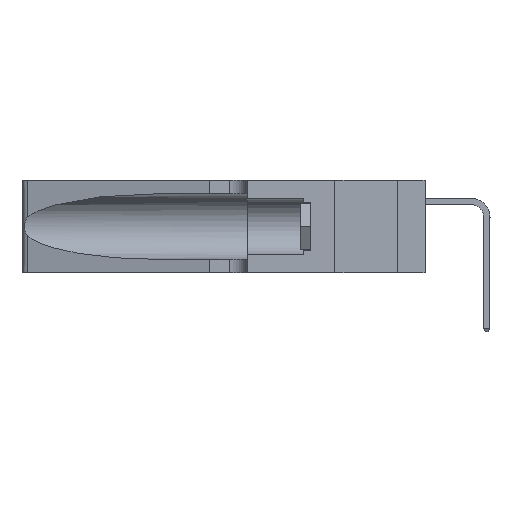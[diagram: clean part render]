
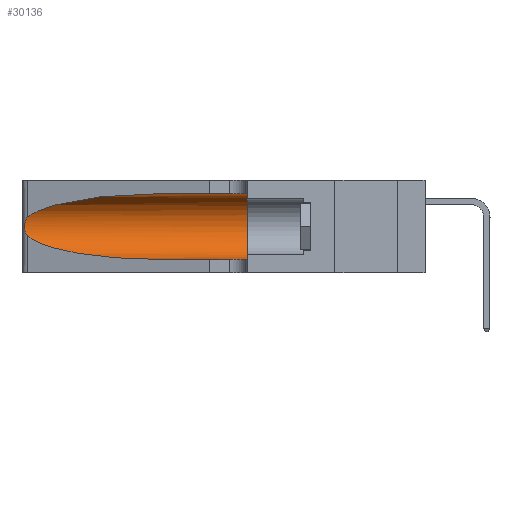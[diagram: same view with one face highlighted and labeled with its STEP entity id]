
A CAD part, left-side view. The second image highlights one B-rep face of the part: STEP entity #30136.
In plain terms, the highlighted cylindrical face has radius 3.308 mm (diameter 6.617 mm), a partial arc.
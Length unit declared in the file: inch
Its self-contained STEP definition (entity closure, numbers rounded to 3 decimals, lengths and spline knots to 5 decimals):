
#444 = CARTESIAN_POINT ( 'NONE',  ( 0.25555, 1.22994, 0.2215 ) ) ;
#615 = CARTESIAN_POINT ( 'NONE',  ( 0.25487, 1.22718, 0.14631 ) ) ;
#868 = VERTEX_POINT ( 'NONE', #48752 ) ;
#929 = DIRECTION ( 'NONE',  ( 0., -1., 0. ) ) ;
#1333 = FACE_OUTER_BOUND ( 'NONE', #9820, .T. ) ;
#1765 = CARTESIAN_POINT ( 'NONE',  ( 0.1305, 0.72297, 0.31525 ) ) ;
#2274 = CARTESIAN_POINT ( 'NONE',  ( 0.1305, 1.61858, 0.31525 ) ) ;
#4525 = CARTESIAN_POINT ( 'NONE',  ( 0.25487, 1.22718, 0.22369 ) ) ;
#4927 = DIRECTION ( 'NONE',  ( 0., -1., 0. ) ) ;
#5170 = ORIENTED_EDGE ( 'NONE', *, *, #38630, .F. ) ;
#5724 = CARTESIAN_POINT ( 'NONE',  ( 0.1305, 0.72297, 0.05475 ) ) ;
#6654 =( BOUNDED_CURVE ( )  B_SPLINE_CURVE ( 3, ( #50206, #21875, #30033, #5724 ),
 .UNSPECIFIED., .F., .F. ) 
 B_SPLINE_CURVE_WITH_KNOTS ( ( 4, 4 ),
 ( 3.44316, 4.71239 ),
 .UNSPECIFIED. ) 
 CURVE ( )  GEOMETRIC_REPRESENTATION_ITEM ( )  RATIONAL_B_SPLINE_CURVE ( ( 1., 0.87, 0.87, 1. ) ) 
 REPRESENTATION_ITEM ( '' )  );
#8615 = CARTESIAN_POINT ( 'NONE',  ( 0.25854, 1.2359, 0.20912 ) ) ;
#9820 = EDGE_LOOP ( 'NONE', ( #46603, #17279, #41911, #24127, #30519, #5170 ) ) ;
#12690 = CARTESIAN_POINT ( 'NONE',  ( 0.26075, 1.23896, 0.19203 ) ) ;
#12732 = CARTESIAN_POINT ( 'NONE',  ( 0.25487, 1.22718, 0.22369 ) ) ;
#14310 = CARTESIAN_POINT ( 'NONE',  ( 0.1305, 0.35, 0.185 ) ) ;
#14736 = CARTESIAN_POINT ( 'NONE',  ( 0.25487, 1.22718, 0.22369 ) ) ;
#16659 = CARTESIAN_POINT ( 'NONE',  ( 0.1305, 0.72297, 0.31525 ) ) ;
#16790 = CARTESIAN_POINT ( 'NONE',  ( 0.26017, 1.23833, 0.17102 ) ) ;
#17021 = VERTEX_POINT ( 'NONE', #27791 ) ;
#17165 = EDGE_CURVE ( 'NONE', #49533, #18717, #21082, .T. ) ;
#17279 = ORIENTED_EDGE ( 'NONE', *, *, #17165, .T. ) ;
#18390 = DIRECTION ( 'NONE',  ( 0., 0., 1. ) ) ;
#18717 = VERTEX_POINT ( 'NONE', #49147 ) ;
#18880 = EDGE_CURVE ( 'NONE', #18717, #28543, #6654, .T. ) ;
#20857 = CARTESIAN_POINT ( 'NONE',  ( 0.25789, 1.23486, 0.15765 ) ) ;
#21082 = B_SPLINE_CURVE_WITH_KNOTS ( 'NONE', 3,
 ( #4525, #444, #28835, #32958, #8615, #36999, #12690, #41062, #16790, #45137, #20857, #49196, #24958, #615 ),
 .UNSPECIFIED., .F., .F.,
 ( 4, 2, 2, 2, 2, 2, 4 ),
 ( 0., 0.00027, 0.00053, 0.00107, 0.0016, 0.00187, 0.00214 ),
 .UNSPECIFIED. ) ;
#21369 = DIRECTION ( 'NONE',  ( 0., 0., -1. ) ) ;
#21875 = CARTESIAN_POINT ( 'NONE',  ( 0.2373, 1.15595, 0.08982 ) ) ;
#24127 = ORIENTED_EDGE ( 'NONE', *, *, #34479, .T. ) ;
#24958 = CARTESIAN_POINT ( 'NONE',  ( 0.25555, 1.22993, 0.14849 ) ) ;
#25184 = CARTESIAN_POINT ( 'NONE',  ( 0.1305, 1.61858, 0.05475 ) ) ;
#27354 = CARTESIAN_POINT ( 'NONE',  ( 0.1305, 0.72297, 0.05475 ) ) ;
#27708 = EDGE_CURVE ( 'NONE', #868, #17021, #36431, .T. ) ;
#27791 = CARTESIAN_POINT ( 'NONE',  ( 0.1305, 0.35, 0.05475 ) ) ;
#28543 = VERTEX_POINT ( 'NONE', #27354 ) ;
#28835 = CARTESIAN_POINT ( 'NONE',  ( 0.25639, 1.23184, 0.21858 ) ) ;
#30033 = CARTESIAN_POINT ( 'NONE',  ( 0.18966, 0.96281, 0.05475 ) ) ;
#30136 = ADVANCED_FACE ( 'NONE', ( #1333 ), #32465, .F. ) ;
#30519 = ORIENTED_EDGE ( 'NONE', *, *, #27708, .F. ) ;
#32465 = CYLINDRICAL_SURFACE ( 'NONE', #32975, 0.13025 ) ;
#32958 = CARTESIAN_POINT ( 'NONE',  ( 0.25787, 1.23484, 0.2124 ) ) ;
#32975 = AXIS2_PLACEMENT_3D ( 'NONE', #45629, #929, #21369 ) ;
#34479 = EDGE_CURVE ( 'NONE', #28543, #17021, #41619, .T. ) ;
#34764 = DIRECTION ( 'NONE',  ( 0., -1., 0. ) ) ;
#36431 = CIRCLE ( 'NONE', #37283, 0.13025 ) ;
#36999 = CARTESIAN_POINT ( 'NONE',  ( 0.26018, 1.23835, 0.19895 ) ) ;
#37035 = CARTESIAN_POINT ( 'NONE',  ( 0.2373, 1.15595, 0.28018 ) ) ;
#37283 = AXIS2_PLACEMENT_3D ( 'NONE', #14310, #42680, #18390 ) ;
#38630 = EDGE_CURVE ( 'NONE', #47607, #868, #45646, .T. ) ;
#39789 =( BOUNDED_CURVE ( )  B_SPLINE_CURVE ( 3, ( #16659, #49061, #37035, #12732 ),
 .UNSPECIFIED., .F., .T. ) 
 B_SPLINE_CURVE_WITH_KNOTS ( ( 4, 4 ),
 ( 1.5708, 2.84003 ),
 .UNSPECIFIED. ) 
 CURVE ( )  GEOMETRIC_REPRESENTATION_ITEM ( )  RATIONAL_B_SPLINE_CURVE ( ( 1., 0.87, 0.87, 1. ) ) 
 REPRESENTATION_ITEM ( '' )  );
#41062 = CARTESIAN_POINT ( 'NONE',  ( 0.26075, 1.23896, 0.178 ) ) ;
#41619 = LINE ( 'NONE', #25184, #42911 ) ;
#41911 = ORIENTED_EDGE ( 'NONE', *, *, #18880, .T. ) ;
#42680 = DIRECTION ( 'NONE',  ( 0., 1., 0. ) ) ;
#42911 = VECTOR ( 'NONE', #4927, 39.37008 ) ;
#44386 = VECTOR ( 'NONE', #34764, 39.37008 ) ;
#45137 = CARTESIAN_POINT ( 'NONE',  ( 0.25856, 1.23593, 0.16098 ) ) ;
#45629 = CARTESIAN_POINT ( 'NONE',  ( 0.1305, 1.61858, 0.185 ) ) ;
#45646 = LINE ( 'NONE', #2274, #44386 ) ;
#46603 = ORIENTED_EDGE ( 'NONE', *, *, #46632, .T. ) ;
#46632 = EDGE_CURVE ( 'NONE', #47607, #49533, #39789, .T. ) ;
#47607 = VERTEX_POINT ( 'NONE', #1765 ) ;
#48752 = CARTESIAN_POINT ( 'NONE',  ( 0.1305, 0.35, 0.31525 ) ) ;
#49061 = CARTESIAN_POINT ( 'NONE',  ( 0.18966, 0.96281, 0.31525 ) ) ;
#49147 = CARTESIAN_POINT ( 'NONE',  ( 0.25487, 1.22718, 0.14631 ) ) ;
#49196 = CARTESIAN_POINT ( 'NONE',  ( 0.25639, 1.23186, 0.15144 ) ) ;
#49533 = VERTEX_POINT ( 'NONE', #14736 ) ;
#50206 = CARTESIAN_POINT ( 'NONE',  ( 0.25487, 1.22718, 0.14631 ) ) ;
